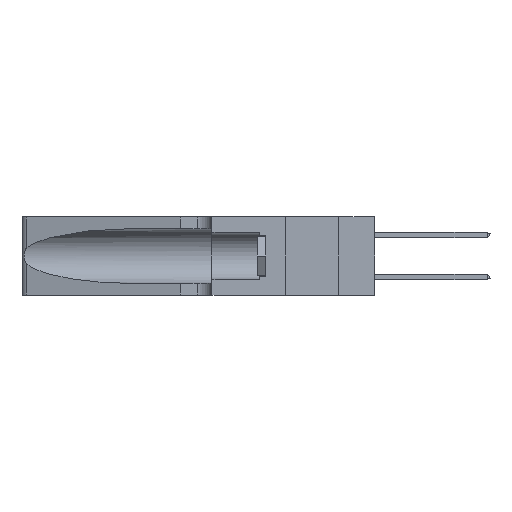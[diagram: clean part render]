
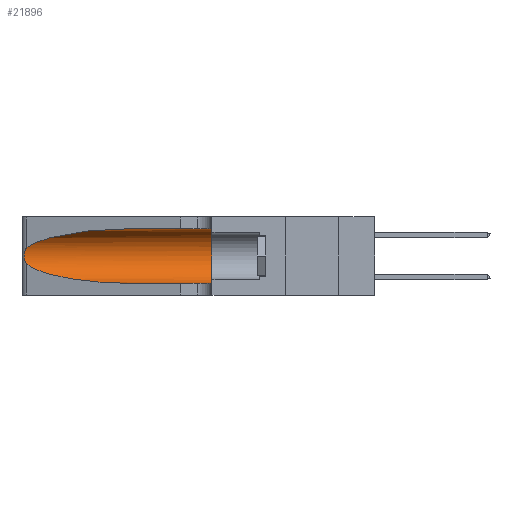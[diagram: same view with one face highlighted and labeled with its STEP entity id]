
A CAD part, left-side view. The second image highlights one B-rep face of the part: STEP entity #21896.
In plain terms, the highlighted cylindrical face has radius 3.308 mm (diameter 6.617 mm), a partial arc.
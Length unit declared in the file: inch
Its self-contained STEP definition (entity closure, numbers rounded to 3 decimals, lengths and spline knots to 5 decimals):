
#244 = ORIENTED_EDGE ( 'NONE', *, *, #13778, .F. ) ;
#379 =( BOUNDED_CURVE ( )  B_SPLINE_CURVE ( 3, ( #642, #13241, #15007, #4347 ),
 .UNSPECIFIED., .F., .F. ) 
 B_SPLINE_CURVE_WITH_KNOTS ( ( 4, 4 ),
 ( 1.5708, 2.84003 ),
 .UNSPECIFIED. ) 
 CURVE ( )  GEOMETRIC_REPRESENTATION_ITEM ( )  RATIONAL_B_SPLINE_CURVE ( ( 1., 0.87, 0.87, 1. ) ) 
 REPRESENTATION_ITEM ( '' )  );
#642 = CARTESIAN_POINT ( 'NONE',  ( 0.1305, 0.72297, 0.31525 ) ) ;
#759 = AXIS2_PLACEMENT_3D ( 'NONE', #14167, #3484, #15895 ) ;
#851 = B_SPLINE_CURVE_WITH_KNOTS ( 'NONE', 3,
 ( #18788, #4715, #13612, #8373, #20527, #10171, #22256, #11941, #1115, #13687, #2982, #15434, #4799, #17160 ),
 .UNSPECIFIED., .F., .F.,
 ( 4, 2, 2, 2, 2, 2, 4 ),
 ( 0., 0.00027, 0.00053, 0.00107, 0.0016, 0.00187, 0.00214 ),
 .UNSPECIFIED. ) ;
#1115 = CARTESIAN_POINT ( 'NONE',  ( 0.26017, 1.23833, 0.17102 ) ) ;
#1887 = VERTEX_POINT ( 'NONE', #18006 ) ;
#2197 = ORIENTED_EDGE ( 'NONE', *, *, #18836, .T. ) ;
#2561 = CIRCLE ( 'NONE', #759, 0.13025 ) ;
#2953 = FACE_OUTER_BOUND ( 'NONE', #13220, .T. ) ;
#2982 = CARTESIAN_POINT ( 'NONE',  ( 0.25789, 1.23486, 0.15765 ) ) ;
#3484 = DIRECTION ( 'NONE',  ( 0., 1., 0. ) ) ;
#3766 = EDGE_CURVE ( 'NONE', #14467, #13222, #851, .T. ) ;
#4049 = LINE ( 'NONE', #7807, #12967 ) ;
#4347 = CARTESIAN_POINT ( 'NONE',  ( 0.25487, 1.22718, 0.22369 ) ) ;
#4412 = CARTESIAN_POINT ( 'NONE',  ( 0.1305, 0.72297, 0.05475 ) ) ;
#4715 = CARTESIAN_POINT ( 'NONE',  ( 0.25555, 1.22994, 0.2215 ) ) ;
#4799 = CARTESIAN_POINT ( 'NONE',  ( 0.25555, 1.22993, 0.14849 ) ) ;
#5184 = EDGE_CURVE ( 'NONE', #17250, #11950, #2561, .T. ) ;
#6129 = EDGE_CURVE ( 'NONE', #1887, #14467, #379, .T. ) ;
#6463 = ORIENTED_EDGE ( 'NONE', *, *, #3766, .T. ) ;
#7153 = CARTESIAN_POINT ( 'NONE',  ( 0.1305, 0.72297, 0.05475 ) ) ;
#7807 = CARTESIAN_POINT ( 'NONE',  ( 0.1305, 1.61858, 0.05475 ) ) ;
#7889 = ORIENTED_EDGE ( 'NONE', *, *, #5184, .F. ) ;
#7998 = CARTESIAN_POINT ( 'NONE',  ( 0.2373, 1.15595, 0.08982 ) ) ;
#8201 = CARTESIAN_POINT ( 'NONE',  ( 0.1305, 1.61858, 0.31525 ) ) ;
#8373 = CARTESIAN_POINT ( 'NONE',  ( 0.25787, 1.23484, 0.2124 ) ) ;
#8398 = VERTEX_POINT ( 'NONE', #7153 ) ;
#10171 = CARTESIAN_POINT ( 'NONE',  ( 0.26018, 1.23835, 0.19895 ) ) ;
#11574 = CARTESIAN_POINT ( 'NONE',  ( 0.25487, 1.22718, 0.14631 ) ) ;
#11941 = CARTESIAN_POINT ( 'NONE',  ( 0.26075, 1.23896, 0.178 ) ) ;
#11948 = CYLINDRICAL_SURFACE ( 'NONE', #21304, 0.13025 ) ;
#11950 = VERTEX_POINT ( 'NONE', #12446 ) ;
#12446 = CARTESIAN_POINT ( 'NONE',  ( 0.1305, 0.35, 0.05475 ) ) ;
#12967 = VECTOR ( 'NONE', #21726, 39.37008 ) ;
#13220 = EDGE_LOOP ( 'NONE', ( #16958, #6463, #2197, #21832, #7889, #244 ) ) ;
#13222 = VERTEX_POINT ( 'NONE', #13855 ) ;
#13241 = CARTESIAN_POINT ( 'NONE',  ( 0.18966, 0.96281, 0.31525 ) ) ;
#13612 = CARTESIAN_POINT ( 'NONE',  ( 0.25639, 1.23184, 0.21858 ) ) ;
#13638 = EDGE_CURVE ( 'NONE', #8398, #11950, #4049, .T. ) ;
#13687 = CARTESIAN_POINT ( 'NONE',  ( 0.25856, 1.23593, 0.16098 ) ) ;
#13778 = EDGE_CURVE ( 'NONE', #1887, #17250, #15442, .T. ) ;
#13855 = CARTESIAN_POINT ( 'NONE',  ( 0.25487, 1.22718, 0.14631 ) ) ;
#14167 = CARTESIAN_POINT ( 'NONE',  ( 0.1305, 0.35, 0.185 ) ) ;
#14467 = VERTEX_POINT ( 'NONE', #17117 ) ;
#15007 = CARTESIAN_POINT ( 'NONE',  ( 0.2373, 1.15595, 0.28018 ) ) ;
#15075 = CARTESIAN_POINT ( 'NONE',  ( 0.18966, 0.96281, 0.05475 ) ) ;
#15434 = CARTESIAN_POINT ( 'NONE',  ( 0.25639, 1.23186, 0.15144 ) ) ;
#15442 = LINE ( 'NONE', #8201, #19452 ) ;
#15895 = DIRECTION ( 'NONE',  ( 0., 0., 1. ) ) ;
#16958 = ORIENTED_EDGE ( 'NONE', *, *, #6129, .T. ) ;
#17117 = CARTESIAN_POINT ( 'NONE',  ( 0.25487, 1.22718, 0.22369 ) ) ;
#17160 = CARTESIAN_POINT ( 'NONE',  ( 0.25487, 1.22718, 0.14631 ) ) ;
#17250 = VERTEX_POINT ( 'NONE', #20650 ) ;
#17539 =( BOUNDED_CURVE ( )  B_SPLINE_CURVE ( 3, ( #11574, #7998, #15075, #4412 ),
 .UNSPECIFIED., .F., .F. ) 
 B_SPLINE_CURVE_WITH_KNOTS ( ( 4, 4 ),
 ( 3.44316, 4.71239 ),
 .UNSPECIFIED. ) 
 CURVE ( )  GEOMETRIC_REPRESENTATION_ITEM ( )  RATIONAL_B_SPLINE_CURVE ( ( 1., 0.87, 0.87, 1. ) ) 
 REPRESENTATION_ITEM ( '' )  );
#18006 = CARTESIAN_POINT ( 'NONE',  ( 0.1305, 0.72297, 0.31525 ) ) ;
#18788 = CARTESIAN_POINT ( 'NONE',  ( 0.25487, 1.22718, 0.22369 ) ) ;
#18836 = EDGE_CURVE ( 'NONE', #13222, #8398, #17539, .T. ) ;
#19452 = VECTOR ( 'NONE', #20353, 39.37008 ) ;
#19498 = CARTESIAN_POINT ( 'NONE',  ( 0.1305, 1.61858, 0.185 ) ) ;
#20353 = DIRECTION ( 'NONE',  ( 0., -1., 0. ) ) ;
#20527 = CARTESIAN_POINT ( 'NONE',  ( 0.25854, 1.2359, 0.20912 ) ) ;
#20650 = CARTESIAN_POINT ( 'NONE',  ( 0.1305, 0.35, 0.31525 ) ) ;
#21242 = DIRECTION ( 'NONE',  ( 0., -1., 0. ) ) ;
#21304 = AXIS2_PLACEMENT_3D ( 'NONE', #19498, #21242, #22878 ) ;
#21726 = DIRECTION ( 'NONE',  ( 0., -1., 0. ) ) ;
#21832 = ORIENTED_EDGE ( 'NONE', *, *, #13638, .T. ) ;
#21896 = ADVANCED_FACE ( 'NONE', ( #2953 ), #11948, .F. ) ;
#22256 = CARTESIAN_POINT ( 'NONE',  ( 0.26075, 1.23896, 0.19203 ) ) ;
#22878 = DIRECTION ( 'NONE',  ( 0., 0., -1. ) ) ;
